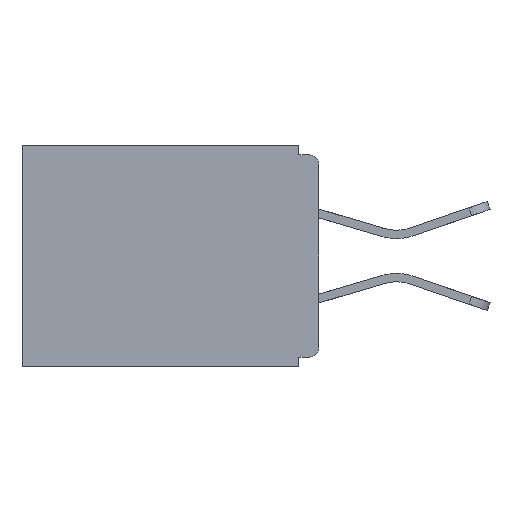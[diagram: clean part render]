
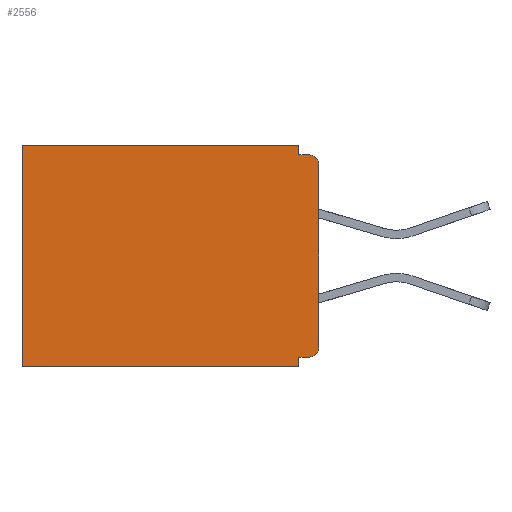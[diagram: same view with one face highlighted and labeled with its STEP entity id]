
A CAD part, left-side view. The second image highlights one B-rep face of the part: STEP entity #2556.
In plain terms, the highlighted planar face has unit normal (-1, 0, 0).
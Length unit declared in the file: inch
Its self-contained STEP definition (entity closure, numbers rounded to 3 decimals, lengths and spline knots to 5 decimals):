
#336 = CARTESIAN_POINT ( 'NONE',  ( 0.298, 0., -0.313 ) ) ;
#373 = ORIENTED_EDGE ( 'NONE', *, *, #2640, .F. ) ;
#480 = CARTESIAN_POINT ( 'NONE',  ( 0.298, 0.031, -0.343 ) ) ;
#513 = ORIENTED_EDGE ( 'NONE', *, *, #5981, .T. ) ;
#616 = DIRECTION ( 'NONE',  ( 0., 0., -1. ) ) ;
#621 = VERTEX_POINT ( 'NONE', #9906 ) ;
#1509 = ORIENTED_EDGE ( 'NONE', *, *, #11424, .F. ) ;
#1860 = CARTESIAN_POINT ( 'NONE',  ( 0.298, 0., -0.015 ) ) ;
#2001 = VERTEX_POINT ( 'NONE', #480 ) ;
#2045 = ORIENTED_EDGE ( 'NONE', *, *, #11534, .T. ) ;
#2453 = DIRECTION ( 'NONE',  ( 0., 1., 0. ) ) ;
#2498 = DIRECTION ( 'NONE',  ( 0., 1., 0. ) ) ;
#2500 = LINE ( 'NONE', #1860, #8371 ) ;
#2556 = ADVANCED_FACE ( 'NONE', ( #2642 ), #10846, .F. ) ;
#2640 = EDGE_CURVE ( 'NONE', #3354, #12452, #2500, .T. ) ;
#2642 = FACE_OUTER_BOUND ( 'NONE', #4796, .T. ) ;
#3010 = CIRCLE ( 'NONE', #5468, 0.015 ) ;
#3330 = DIRECTION ( 'NONE',  ( 0., 0., -1. ) ) ;
#3354 = VERTEX_POINT ( 'NONE', #8999 ) ;
#3387 = AXIS2_PLACEMENT_3D ( 'NONE', #11552, #11668, #8556 ) ;
#3459 = DIRECTION ( 'NONE',  ( 0., 0., -1. ) ) ;
#3478 = CARTESIAN_POINT ( 'NONE',  ( 0.298, 0., 0. ) ) ;
#3783 = VECTOR ( 'NONE', #4631, 39.37008 ) ;
#3861 = ORIENTED_EDGE ( 'NONE', *, *, #8391, .F. ) ;
#3949 = ORIENTED_EDGE ( 'NONE', *, *, #7093, .F. ) ;
#3955 = CARTESIAN_POINT ( 'NONE',  ( 0.298, 0.031, -0.328 ) ) ;
#4028 = DIRECTION ( 'NONE',  ( 0., -1., 0. ) ) ;
#4050 = DIRECTION ( 'NONE',  ( 0., 0., -1. ) ) ;
#4069 = VECTOR ( 'NONE', #2453, 39.37008 ) ;
#4075 = VECTOR ( 'NONE', #2498, 39.37008 ) ;
#4434 = CARTESIAN_POINT ( 'NONE',  ( 0.298, 0.015, -0.015 ) ) ;
#4631 = DIRECTION ( 'NONE',  ( 0., 0., -1. ) ) ;
#4796 = EDGE_LOOP ( 'NONE', ( #2045, #373, #3949, #4965, #10535, #11934, #6960, #3861, #513, #1509 ) ) ;
#4965 = ORIENTED_EDGE ( 'NONE', *, *, #9627, .T. ) ;
#5343 = VECTOR ( 'NONE', #3330, 39.37008 ) ;
#5377 = DIRECTION ( 'NONE',  ( -1., 0., 0. ) ) ;
#5468 = AXIS2_PLACEMENT_3D ( 'NONE', #6463, #5377, #3459 ) ;
#5738 = DIRECTION ( 'NONE',  ( 0., 1., 0. ) ) ;
#5981 = EDGE_CURVE ( 'NONE', #10507, #11197, #3010, .T. ) ;
#6165 = VECTOR ( 'NONE', #12304, 39.37008 ) ;
#6227 = EDGE_CURVE ( 'NONE', #6717, #2001, #9203, .T. ) ;
#6326 = LINE ( 'NONE', #10308, #6165 ) ;
#6365 = VERTEX_POINT ( 'NONE', #10304 ) ;
#6463 = CARTESIAN_POINT ( 'NONE',  ( 0.298, 0.015, -0.313 ) ) ;
#6498 = LINE ( 'NONE', #9648, #3783 ) ;
#6590 = LINE ( 'NONE', #12310, #5343 ) ;
#6637 = EDGE_CURVE ( 'NONE', #2001, #12563, #6787, .T. ) ;
#6639 = VECTOR ( 'NONE', #4050, 39.37008 ) ;
#6717 = VERTEX_POINT ( 'NONE', #3955 ) ;
#6757 = CARTESIAN_POINT ( 'NONE',  ( 0.298, 0., -0.343 ) ) ;
#6782 = LINE ( 'NONE', #3478, #4075 ) ;
#6787 = LINE ( 'NONE', #6757, #12509 ) ;
#6960 = ORIENTED_EDGE ( 'NONE', *, *, #6227, .F. ) ;
#7093 = EDGE_CURVE ( 'NONE', #11426, #3354, #6498, .T. ) ;
#7133 = AXIS2_PLACEMENT_3D ( 'NONE', #11891, #11730, #616 ) ;
#7400 = CARTESIAN_POINT ( 'NONE',  ( 0.298, 0.031, 0. ) ) ;
#7546 = EDGE_CURVE ( 'NONE', #6365, #12563, #6326, .T. ) ;
#7751 = CARTESIAN_POINT ( 'NONE',  ( 0.298, 0.46, -0.343 ) ) ;
#8371 = VECTOR ( 'NONE', #4028, 39.37008 ) ;
#8391 = EDGE_CURVE ( 'NONE', #10507, #6717, #11203, .T. ) ;
#8556 = DIRECTION ( 'NONE',  ( 0., 0., -1. ) ) ;
#8999 = CARTESIAN_POINT ( 'NONE',  ( 0.298, 0.031, -0.015 ) ) ;
#9203 = LINE ( 'NONE', #10029, #6639 ) ;
#9232 = CARTESIAN_POINT ( 'NONE',  ( 0.298, 0.015, -0.328 ) ) ;
#9627 = EDGE_CURVE ( 'NONE', #11426, #6365, #6782, .T. ) ;
#9648 = CARTESIAN_POINT ( 'NONE',  ( 0.298, 0.031, -0.343 ) ) ;
#9906 = CARTESIAN_POINT ( 'NONE',  ( 0.298, 0., -0.03 ) ) ;
#10029 = CARTESIAN_POINT ( 'NONE',  ( 0.298, 0.031, -0.343 ) ) ;
#10304 = CARTESIAN_POINT ( 'NONE',  ( 0.298, 0.46, 0. ) ) ;
#10308 = CARTESIAN_POINT ( 'NONE',  ( 0.298, 0.46, 0. ) ) ;
#10507 = VERTEX_POINT ( 'NONE', #9232 ) ;
#10535 = ORIENTED_EDGE ( 'NONE', *, *, #7546, .T. ) ;
#10846 = PLANE ( 'NONE',  #7133 ) ;
#11197 = VERTEX_POINT ( 'NONE', #336 ) ;
#11203 = LINE ( 'NONE', #12511, #4069 ) ;
#11424 = EDGE_CURVE ( 'NONE', #621, #11197, #6590, .T. ) ;
#11426 = VERTEX_POINT ( 'NONE', #7400 ) ;
#11534 = EDGE_CURVE ( 'NONE', #621, #12452, #11954, .T. ) ;
#11552 = CARTESIAN_POINT ( 'NONE',  ( 0.298, 0.015, -0.03 ) ) ;
#11668 = DIRECTION ( 'NONE',  ( -1., 0., 0. ) ) ;
#11730 = DIRECTION ( 'NONE',  ( 1., 0., 0. ) ) ;
#11891 = CARTESIAN_POINT ( 'NONE',  ( 0.298, 0., 0. ) ) ;
#11934 = ORIENTED_EDGE ( 'NONE', *, *, #6637, .F. ) ;
#11954 = CIRCLE ( 'NONE', #3387, 0.015 ) ;
#12304 = DIRECTION ( 'NONE',  ( 0., 0., -1. ) ) ;
#12310 = CARTESIAN_POINT ( 'NONE',  ( 0.298, 0., 0. ) ) ;
#12452 = VERTEX_POINT ( 'NONE', #4434 ) ;
#12509 = VECTOR ( 'NONE', #5738, 39.37008 ) ;
#12511 = CARTESIAN_POINT ( 'NONE',  ( 0.298, 0., -0.328 ) ) ;
#12563 = VERTEX_POINT ( 'NONE', #7751 ) ;
